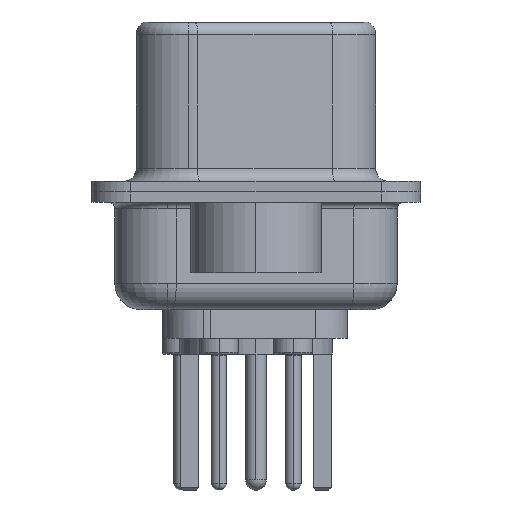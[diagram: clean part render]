
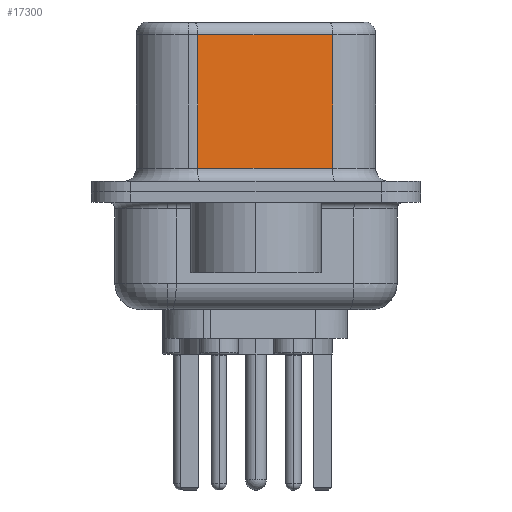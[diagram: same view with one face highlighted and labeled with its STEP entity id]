
A CAD part, left-side view. The second image highlights one B-rep face of the part: STEP entity #17300.
In plain terms, the highlighted planar face has unit normal (-0.985, -0.174, 0).
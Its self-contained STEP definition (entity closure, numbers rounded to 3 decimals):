
#1320 = EDGE_CURVE ( 'NONE', #5232, #19607, #7579, .T. ) ;
#1538 = ORIENTED_EDGE ( 'NONE', *, *, #1320, .T. ) ;
#2406 = DIRECTION ( 'NONE',  ( 0., 0., -1. ) ) ;
#3416 = CARTESIAN_POINT ( 'NONE',  ( 4.585, -2.927, 0.9 ) ) ;
#3800 = CARTESIAN_POINT ( 'NONE',  ( 4.585, -2.927, 6.02 ) ) ;
#4537 = ORIENTED_EDGE ( 'NONE', *, *, #7603, .T. ) ;
#5066 = VECTOR ( 'NONE', #10563, 1000. ) ;
#5232 = VERTEX_POINT ( 'NONE', #3800 ) ;
#6113 = LINE ( 'NONE', #12772, #22115 ) ;
#7434 = ORIENTED_EDGE ( 'NONE', *, *, #14879, .T. ) ;
#7579 = LINE ( 'NONE', #18184, #5066 ) ;
#7603 = EDGE_CURVE ( 'NONE', #19607, #20024, #6113, .T. ) ;
#7758 = LINE ( 'NONE', #3416, #16179 ) ;
#8618 = FACE_OUTER_BOUND ( 'NONE', #10690, .T. ) ;
#8621 = CARTESIAN_POINT ( 'NONE',  ( 3.675, 2.233, 0.9 ) ) ;
#9957 = AXIS2_PLACEMENT_3D ( 'NONE', #24185, #14606, #14769 ) ;
#10445 = VECTOR ( 'NONE', #18241, 1000. ) ;
#10563 = DIRECTION ( 'NONE',  ( -0.174, 0.985, 0. ) ) ;
#10690 = EDGE_LOOP ( 'NONE', ( #15409, #1538, #4537, #7434 ) ) ;
#11068 = LINE ( 'NONE', #24111, #10445 ) ;
#12772 = CARTESIAN_POINT ( 'NONE',  ( 3.675, 2.233, 6.52 ) ) ;
#12890 = VERTEX_POINT ( 'NONE', #16621 ) ;
#13328 = CARTESIAN_POINT ( 'NONE',  ( 3.675, 2.233, 6.02 ) ) ;
#14606 = DIRECTION ( 'NONE',  ( 0.985, 0.174, 0. ) ) ;
#14769 = DIRECTION ( 'NONE',  ( -0.174, 0.985, 0. ) ) ;
#14879 = EDGE_CURVE ( 'NONE', #20024, #12890, #7758, .T. ) ;
#15409 = ORIENTED_EDGE ( 'NONE', *, *, #17922, .F. ) ;
#16179 = VECTOR ( 'NONE', #21124, 1000. ) ;
#16621 = CARTESIAN_POINT ( 'NONE',  ( 4.585, -2.927, 0.9 ) ) ;
#17300 = ADVANCED_FACE ( 'NONE', ( #8618 ), #24273, .F. ) ;
#17922 = EDGE_CURVE ( 'NONE', #5232, #12890, #11068, .T. ) ;
#18184 = CARTESIAN_POINT ( 'NONE',  ( 4.585, -2.927, 6.02 ) ) ;
#18241 = DIRECTION ( 'NONE',  ( 0., 0., -1. ) ) ;
#19607 = VERTEX_POINT ( 'NONE', #13328 ) ;
#20024 = VERTEX_POINT ( 'NONE', #8621 ) ;
#21124 = DIRECTION ( 'NONE',  ( 0.174, -0.985, 0. ) ) ;
#22115 = VECTOR ( 'NONE', #2406, 1000. ) ;
#24111 = CARTESIAN_POINT ( 'NONE',  ( 4.585, -2.927, 6.52 ) ) ;
#24185 = CARTESIAN_POINT ( 'NONE',  ( 4.585, -2.927, 6.52 ) ) ;
#24273 = PLANE ( 'NONE',  #9957 ) ;
